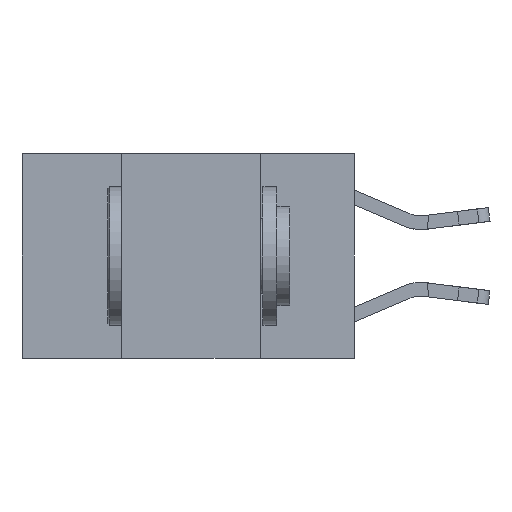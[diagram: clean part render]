
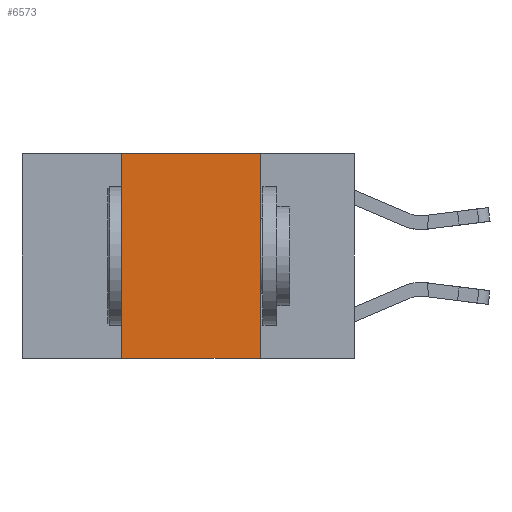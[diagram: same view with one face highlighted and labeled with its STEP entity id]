
A CAD part, left-side view. The second image highlights one B-rep face of the part: STEP entity #6573.
In plain terms, the highlighted planar face has unit normal (-1, 0, 0).
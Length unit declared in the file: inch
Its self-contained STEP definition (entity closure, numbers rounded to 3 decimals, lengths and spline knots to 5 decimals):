
#252 = AXIS2_PLACEMENT_3D ( 'NONE', #14155, #16330, #3368 ) ;
#1468 = VECTOR ( 'NONE', #13940, 39.37008 ) ;
#1507 = VERTEX_POINT ( 'NONE', #15896 ) ;
#1617 = VERTEX_POINT ( 'NONE', #5476 ) ;
#2112 = VERTEX_POINT ( 'NONE', #6891 ) ;
#2987 = EDGE_CURVE ( 'NONE', #2112, #1507, #20488, .T. ) ;
#3368 = DIRECTION ( 'NONE',  ( 0., 0., -1. ) ) ;
#3657 = ORIENTED_EDGE ( 'NONE', *, *, #2987, .F. ) ;
#4166 = VERTEX_POINT ( 'NONE', #17266 ) ;
#4371 = DIRECTION ( 'NONE',  ( 0., -1., 0. ) ) ;
#5476 = CARTESIAN_POINT ( 'NONE',  ( 0., 0.17, -0.37 ) ) ;
#6528 = ORIENTED_EDGE ( 'NONE', *, *, #11023, .F. ) ;
#6573 = ADVANCED_FACE ( 'NONE', ( #14919 ), #27044, .F. ) ;
#6891 = CARTESIAN_POINT ( 'NONE',  ( 0., 0.42, -0.37 ) ) ;
#7947 = LINE ( 'NONE', #22549, #1468 ) ;
#9389 = ORIENTED_EDGE ( 'NONE', *, *, #10815, .F. ) ;
#10089 = DIRECTION ( 'NONE',  ( 0., 0., 1. ) ) ;
#10447 = LINE ( 'NONE', #15173, #21280 ) ;
#10815 = EDGE_CURVE ( 'NONE', #4166, #1617, #7947, .T. ) ;
#11023 = EDGE_CURVE ( 'NONE', #1507, #4166, #19070, .T. ) ;
#12441 = DIRECTION ( 'NONE',  ( 0., -1., 0. ) ) ;
#13940 = DIRECTION ( 'NONE',  ( 0., 0., -1. ) ) ;
#14155 = CARTESIAN_POINT ( 'NONE',  ( 0., 0.6, 0. ) ) ;
#14224 = ORIENTED_EDGE ( 'NONE', *, *, #23839, .T. ) ;
#14919 = FACE_OUTER_BOUND ( 'NONE', #23034, .T. ) ;
#15173 = CARTESIAN_POINT ( 'NONE',  ( 0., 0.6, -0.37 ) ) ;
#15896 = CARTESIAN_POINT ( 'NONE',  ( 0., 0.42, 0. ) ) ;
#16330 = DIRECTION ( 'NONE',  ( 1., 0., 0. ) ) ;
#17266 = CARTESIAN_POINT ( 'NONE',  ( 0., 0.17, 0. ) ) ;
#19070 = LINE ( 'NONE', #27509, #24125 ) ;
#20488 = LINE ( 'NONE', #27319, #25526 ) ;
#21280 = VECTOR ( 'NONE', #4371, 39.37008 ) ;
#22549 = CARTESIAN_POINT ( 'NONE',  ( 0., 0.17, 0. ) ) ;
#23034 = EDGE_LOOP ( 'NONE', ( #9389, #6528, #3657, #14224 ) ) ;
#23839 = EDGE_CURVE ( 'NONE', #2112, #1617, #10447, .T. ) ;
#24125 = VECTOR ( 'NONE', #12441, 39.37008 ) ;
#25526 = VECTOR ( 'NONE', #10089, 39.37008 ) ;
#27044 = PLANE ( 'NONE',  #252 ) ;
#27319 = CARTESIAN_POINT ( 'NONE',  ( 0., 0.42, 0. ) ) ;
#27509 = CARTESIAN_POINT ( 'NONE',  ( 0., 0.6, 0. ) ) ;
